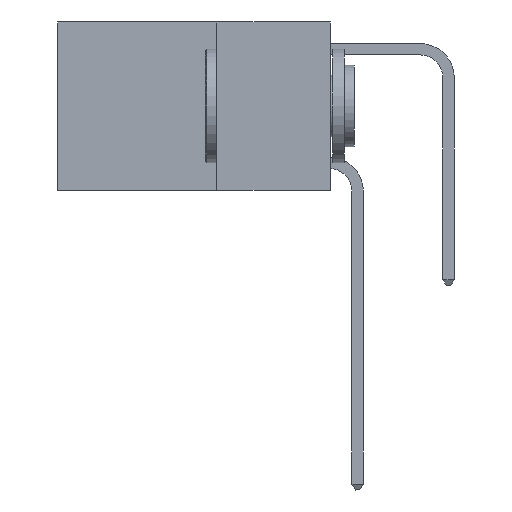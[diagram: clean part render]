
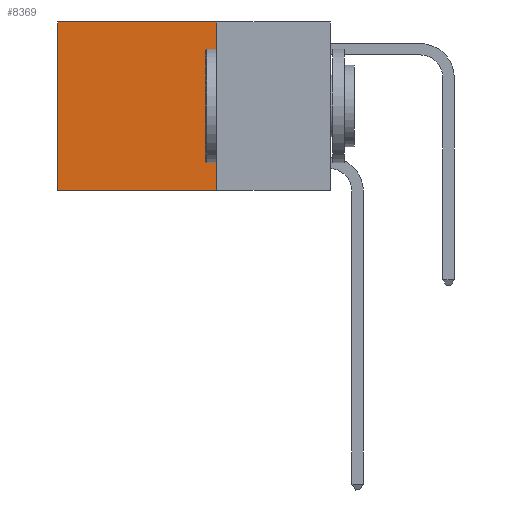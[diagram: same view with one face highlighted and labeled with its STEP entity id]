
A CAD part, left-side view. The second image highlights one B-rep face of the part: STEP entity #8369.
In plain terms, the highlighted planar face has unit normal (-1, 0, 0).
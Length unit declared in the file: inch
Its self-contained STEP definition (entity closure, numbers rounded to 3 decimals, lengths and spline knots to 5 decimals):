
#48 = ORIENTED_EDGE ( 'NONE', *, *, #9929, .T. ) ;
#357 = CARTESIAN_POINT ( 'NONE',  ( 0.2625, 0.6, 0. ) ) ;
#573 = DIRECTION ( 'NONE',  ( 0., 0., -1. ) ) ;
#800 = ORIENTED_EDGE ( 'NONE', *, *, #9141, .T. ) ;
#827 = LINE ( 'NONE', #11187, #5106 ) ;
#1491 = VERTEX_POINT ( 'NONE', #10718 ) ;
#1542 = CARTESIAN_POINT ( 'NONE',  ( 0.2625, 0.6, 0. ) ) ;
#1861 = AXIS2_PLACEMENT_3D ( 'NONE', #9227, #11113, #8394 ) ;
#1962 = VECTOR ( 'NONE', #8321, 39.37008 ) ;
#2080 = CARTESIAN_POINT ( 'NONE',  ( 0.2625, 0.25, 0. ) ) ;
#2081 = VECTOR ( 'NONE', #573, 39.37008 ) ;
#2493 = DIRECTION ( 'NONE',  ( 0., 1., 0. ) ) ;
#2955 = ORIENTED_EDGE ( 'NONE', *, *, #4664, .F. ) ;
#4625 = LINE ( 'NONE', #357, #2081 ) ;
#4664 = EDGE_CURVE ( 'NONE', #8468, #5241, #4682, .T. ) ;
#4682 = LINE ( 'NONE', #2080, #1962 ) ;
#5106 = VECTOR ( 'NONE', #2493, 39.37008 ) ;
#5241 = VERTEX_POINT ( 'NONE', #6384 ) ;
#5693 = VECTOR ( 'NONE', #7736, 39.37008 ) ;
#6171 = CARTESIAN_POINT ( 'NONE',  ( 0.2625, 0.25, 0. ) ) ;
#6384 = CARTESIAN_POINT ( 'NONE',  ( 0.2625, 0.25, -0.37 ) ) ;
#6688 = FACE_OUTER_BOUND ( 'NONE', #8430, .T. ) ;
#6715 = VERTEX_POINT ( 'NONE', #1542 ) ;
#7519 = ORIENTED_EDGE ( 'NONE', *, *, #10549, .F. ) ;
#7641 = PLANE ( 'NONE',  #1861 ) ;
#7736 = DIRECTION ( 'NONE',  ( 0., 1., 0. ) ) ;
#8321 = DIRECTION ( 'NONE',  ( 0., 0., -1. ) ) ;
#8369 = ADVANCED_FACE ( 'NONE', ( #6688 ), #7641, .F. ) ;
#8394 = DIRECTION ( 'NONE',  ( 0., 0., -1. ) ) ;
#8430 = EDGE_LOOP ( 'NONE', ( #48, #7519, #2955, #800 ) ) ;
#8468 = VERTEX_POINT ( 'NONE', #6171 ) ;
#8637 = LINE ( 'NONE', #8747, #5693 ) ;
#8747 = CARTESIAN_POINT ( 'NONE',  ( 0.2625, 0.25, -0.37 ) ) ;
#9141 = EDGE_CURVE ( 'NONE', #8468, #6715, #827, .T. ) ;
#9227 = CARTESIAN_POINT ( 'NONE',  ( 0.2625, 0.25, 0. ) ) ;
#9929 = EDGE_CURVE ( 'NONE', #6715, #1491, #4625, .T. ) ;
#10549 = EDGE_CURVE ( 'NONE', #5241, #1491, #8637, .T. ) ;
#10718 = CARTESIAN_POINT ( 'NONE',  ( 0.2625, 0.6, -0.37 ) ) ;
#11113 = DIRECTION ( 'NONE',  ( 1., 0., 0. ) ) ;
#11187 = CARTESIAN_POINT ( 'NONE',  ( 0.2625, 0.25, 0. ) ) ;
